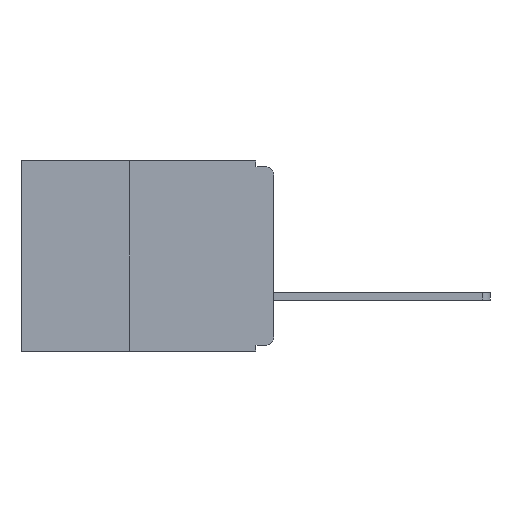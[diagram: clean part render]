
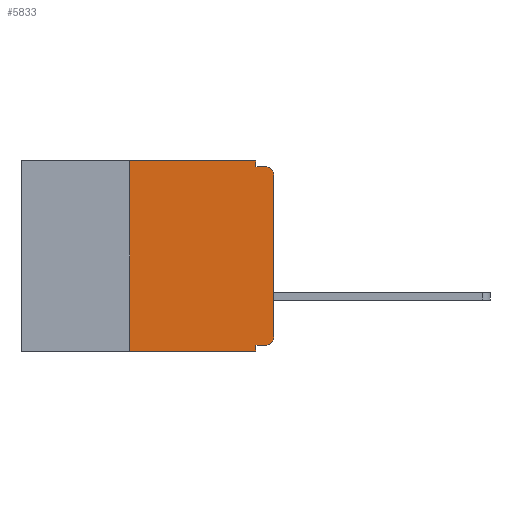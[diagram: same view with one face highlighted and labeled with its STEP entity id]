
A CAD part, left-side view. The second image highlights one B-rep face of the part: STEP entity #5833.
In plain terms, the highlighted planar face has unit normal (-1, 0, 0).
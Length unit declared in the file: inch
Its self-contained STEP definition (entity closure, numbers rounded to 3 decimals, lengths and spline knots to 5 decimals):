
#47 = CARTESIAN_POINT ( 'NONE',  ( 0., 0.031, -0.01 ) ) ;
#612 = EDGE_CURVE ( 'NONE', #15101, #13644, #11307, .T. ) ;
#652 = EDGE_CURVE ( 'NONE', #10577, #2597, #9658, .T. ) ;
#674 = EDGE_CURVE ( 'NONE', #10577, #8506, #9574, .T. ) ;
#764 = EDGE_CURVE ( 'NONE', #10746, #8506, #7813, .T. ) ;
#1178 = ORIENTED_EDGE ( 'NONE', *, *, #15014, .T. ) ;
#1246 = ORIENTED_EDGE ( 'NONE', *, *, #12443, .T. ) ;
#1334 = ORIENTED_EDGE ( 'NONE', *, *, #8942, .F. ) ;
#1533 = ORIENTED_EDGE ( 'NONE', *, *, #612, .F. ) ;
#1661 = ORIENTED_EDGE ( 'NONE', *, *, #15775, .F. ) ;
#1679 = ORIENTED_EDGE ( 'NONE', *, *, #652, .F. ) ;
#1822 = ORIENTED_EDGE ( 'NONE', *, *, #674, .T. ) ;
#2046 = VECTOR ( 'NONE', #2623, 39.37008 ) ;
#2086 = CARTESIAN_POINT ( 'NONE',  ( 0., 0.031, 0. ) ) ;
#2107 = CARTESIAN_POINT ( 'NONE',  ( 0., 0.437, 0. ) ) ;
#2113 = ORIENTED_EDGE ( 'NONE', *, *, #764, .F. ) ;
#2155 = LINE ( 'NONE', #2107, #2046 ) ;
#2251 = ORIENTED_EDGE ( 'NONE', *, *, #12760, .F. ) ;
#2272 = ORIENTED_EDGE ( 'NONE', *, *, #16685, .T. ) ;
#2597 = VERTEX_POINT ( 'NONE', #9523 ) ;
#2623 = DIRECTION ( 'NONE',  ( 0., -1., 0. ) ) ;
#3313 = VERTEX_POINT ( 'NONE', #3659 ) ;
#3659 = CARTESIAN_POINT ( 'NONE',  ( 0., 0.015, -0.01 ) ) ;
#5833 = ADVANCED_FACE ( 'NONE', ( #15243 ), #7774, .F. ) ;
#6150 = AXIS2_PLACEMENT_3D ( 'NONE', #8378, #7713, #7499 ) ;
#6464 = LINE ( 'NONE', #14624, #6519 ) ;
#6519 = VECTOR ( 'NONE', #14520, 39.37008 ) ;
#7469 = VECTOR ( 'NONE', #15064, 39.37008 ) ;
#7499 = DIRECTION ( 'NONE',  ( 0., 0., -1. ) ) ;
#7713 = DIRECTION ( 'NONE',  ( 1., 0., 0. ) ) ;
#7774 = PLANE ( 'NONE',  #6150 ) ;
#7813 = LINE ( 'NONE', #10267, #7469 ) ;
#7856 = VERTEX_POINT ( 'NONE', #8943 ) ;
#7871 = DIRECTION ( 'NONE',  ( 0., 0., -1. ) ) ;
#8332 = CARTESIAN_POINT ( 'NONE',  ( 0., 0.437, -0.33 ) ) ;
#8378 = CARTESIAN_POINT ( 'NONE',  ( 0., 0.437, 0. ) ) ;
#8396 = DIRECTION ( 'NONE',  ( 0., -1., 0. ) ) ;
#8506 = VERTEX_POINT ( 'NONE', #14844 ) ;
#8794 = VECTOR ( 'NONE', #8396, 39.37008 ) ;
#8801 = AXIS2_PLACEMENT_3D ( 'NONE', #9367, #9624, #9564 ) ;
#8843 = VERTEX_POINT ( 'NONE', #18032 ) ;
#8942 = EDGE_CURVE ( 'NONE', #13644, #3313, #11578, .T. ) ;
#8943 = CARTESIAN_POINT ( 'NONE',  ( 0., 0., -0.025 ) ) ;
#9367 = CARTESIAN_POINT ( 'NONE',  ( 0., 0.015, -0.025 ) ) ;
#9523 = CARTESIAN_POINT ( 'NONE',  ( 0., 0.25, 0. ) ) ;
#9564 = DIRECTION ( 'NONE',  ( 0., 0., -1. ) ) ;
#9574 = LINE ( 'NONE', #8332, #8794 ) ;
#9624 = DIRECTION ( 'NONE',  ( -1., 0., 0. ) ) ;
#9658 = LINE ( 'NONE', #12545, #9675 ) ;
#9675 = VECTOR ( 'NONE', #14045, 39.37008 ) ;
#10235 = VERTEX_POINT ( 'NONE', #17454 ) ;
#10253 = CARTESIAN_POINT ( 'NONE',  ( 0., 0.031, 0. ) ) ;
#10267 = CARTESIAN_POINT ( 'NONE',  ( 0., 0.031, -0.33 ) ) ;
#10577 = VERTEX_POINT ( 'NONE', #18086 ) ;
#10746 = VERTEX_POINT ( 'NONE', #14316 ) ;
#11307 = LINE ( 'NONE', #2086, #12539 ) ;
#11559 = VECTOR ( 'NONE', #14731, 39.37008 ) ;
#11578 = LINE ( 'NONE', #14955, #11559 ) ;
#12443 = EDGE_CURVE ( 'NONE', #7856, #3313, #17517, .T. ) ;
#12539 = VECTOR ( 'NONE', #7871, 39.37008 ) ;
#12545 = CARTESIAN_POINT ( 'NONE',  ( 0., 0.25, -0.33 ) ) ;
#12760 = EDGE_CURVE ( 'NONE', #8843, #10746, #16282, .T. ) ;
#12834 = AXIS2_PLACEMENT_3D ( 'NONE', #13848, #13713, #13510 ) ;
#13510 = DIRECTION ( 'NONE',  ( 0., 0., -1. ) ) ;
#13644 = VERTEX_POINT ( 'NONE', #47 ) ;
#13713 = DIRECTION ( 'NONE',  ( -1., 0., 0. ) ) ;
#13848 = CARTESIAN_POINT ( 'NONE',  ( 0., 0.015, -0.305 ) ) ;
#14045 = DIRECTION ( 'NONE',  ( 0., 0., 1. ) ) ;
#14316 = CARTESIAN_POINT ( 'NONE',  ( 0., 0.031, -0.32 ) ) ;
#14520 = DIRECTION ( 'NONE',  ( 0., 0., 1. ) ) ;
#14624 = CARTESIAN_POINT ( 'NONE',  ( 0., 0., 0. ) ) ;
#14731 = DIRECTION ( 'NONE',  ( 0., -1., 0. ) ) ;
#14844 = CARTESIAN_POINT ( 'NONE',  ( 0., 0.031, -0.33 ) ) ;
#14955 = CARTESIAN_POINT ( 'NONE',  ( 0., 0., -0.01 ) ) ;
#15014 = EDGE_CURVE ( 'NONE', #10235, #7856, #6464, .T. ) ;
#15064 = DIRECTION ( 'NONE',  ( 0., 0., -1. ) ) ;
#15101 = VERTEX_POINT ( 'NONE', #10253 ) ;
#15243 = FACE_OUTER_BOUND ( 'NONE', #16704, .T. ) ;
#15718 = CIRCLE ( 'NONE', #12834, 0.015 ) ;
#15775 = EDGE_CURVE ( 'NONE', #2597, #15101, #2155, .T. ) ;
#16210 = VECTOR ( 'NONE', #16334, 39.37008 ) ;
#16282 = LINE ( 'NONE', #16382, #16210 ) ;
#16334 = DIRECTION ( 'NONE',  ( 0., 1., 0. ) ) ;
#16382 = CARTESIAN_POINT ( 'NONE',  ( 0., 0., -0.32 ) ) ;
#16685 = EDGE_CURVE ( 'NONE', #8843, #10235, #15718, .T. ) ;
#16704 = EDGE_LOOP ( 'NONE', ( #1178, #1246, #1334, #1533, #1661, #1679, #1822, #2113, #2251, #2272 ) ) ;
#17454 = CARTESIAN_POINT ( 'NONE',  ( 0., 0., -0.305 ) ) ;
#17517 = CIRCLE ( 'NONE', #8801, 0.015 ) ;
#18032 = CARTESIAN_POINT ( 'NONE',  ( 0., 0.015, -0.32 ) ) ;
#18086 = CARTESIAN_POINT ( 'NONE',  ( 0., 0.25, -0.33 ) ) ;
